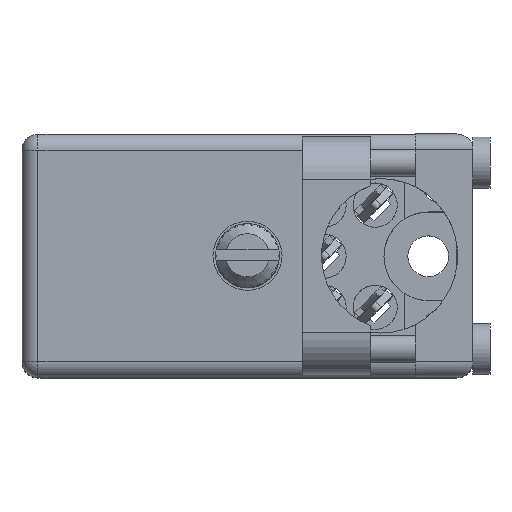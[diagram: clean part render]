
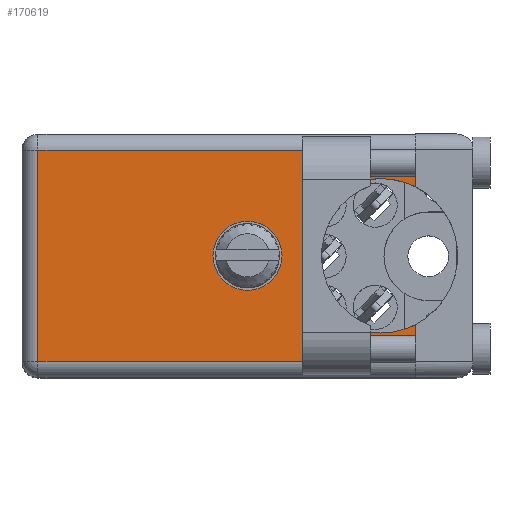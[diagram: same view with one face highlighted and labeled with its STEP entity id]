
A CAD part, top view. The second image highlights one B-rep face of the part: STEP entity #170619.
In plain terms, the highlighted face is planar.
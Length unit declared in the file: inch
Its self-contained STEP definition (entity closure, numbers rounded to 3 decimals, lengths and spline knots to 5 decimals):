
#3561 = AXIS2_PLACEMENT_3D ( 'NONE', #135737, #51711, #151351 ) ;
#6089 = ORIENTED_EDGE ( 'NONE', *, *, #53595, .F. ) ;
#8694 = LINE ( 'NONE', #50967, #156568 ) ;
#12902 = VECTOR ( 'NONE', #153332, 39.37008 ) ;
#13545 = ORIENTED_EDGE ( 'NONE', *, *, #129859, .F. ) ;
#19530 = CARTESIAN_POINT ( 'NONE',  ( 1.155, 0.906, -0.047 ) ) ;
#21340 = DIRECTION ( 'NONE',  ( 0., 1., 0. ) ) ;
#23151 = ORIENTED_EDGE ( 'NONE', *, *, #174199, .F. ) ;
#28073 = DIRECTION ( 'NONE',  ( 0., 0., 1. ) ) ;
#28147 = CARTESIAN_POINT ( 'NONE',  ( 1.155, 0.906, -0.047 ) ) ;
#28583 = AXIS2_PLACEMENT_3D ( 'NONE', #70898, #29603, #142340 ) ;
#29059 = DIRECTION ( 'NONE',  ( 0., 0., 1. ) ) ;
#29271 = CARTESIAN_POINT ( 'NONE',  ( 0.047, 0.906, -0.668 ) ) ;
#29603 = DIRECTION ( 'NONE',  ( 0., 1., 0. ) ) ;
#30458 = VERTEX_POINT ( 'NONE', #82985 ) ;
#31246 = AXIS2_PLACEMENT_3D ( 'NONE', #133064, #129263, #29059 ) ;
#33281 = DIRECTION ( 'NONE',  ( 0., 0., 1. ) ) ;
#36613 = DIRECTION ( 'NONE',  ( -1., 0., 0. ) ) ;
#39174 = EDGE_CURVE ( 'NONE', #137315, #173928, #170800, .T. ) ;
#39487 = LINE ( 'NONE', #28147, #147174 ) ;
#40610 = ORIENTED_EDGE ( 'NONE', *, *, #67839, .T. ) ;
#42143 = CIRCLE ( 'NONE', #3561, 0.1015 ) ;
#45993 = DIRECTION ( 'NONE',  ( 0., 0., 1. ) ) ;
#46814 = DIRECTION ( 'NONE',  ( 1., 0., 0. ) ) ;
#48871 = ORIENTED_EDGE ( 'NONE', *, *, #39174, .F. ) ;
#50967 = CARTESIAN_POINT ( 'NONE',  ( 0., 0.906, -0.668 ) ) ;
#51079 = AXIS2_PLACEMENT_3D ( 'NONE', #106501, #21340, #105235 ) ;
#51711 = DIRECTION ( 'NONE',  ( 0., 1., 0. ) ) ;
#53595 = EDGE_CURVE ( 'NONE', #85711, #162808, #42143, .T. ) ;
#54679 = EDGE_CURVE ( 'NONE', #141181, #30458, #125060, .T. ) ;
#54695 = CARTESIAN_POINT ( 'NONE',  ( 1.155, 0.906, 0. ) ) ;
#56258 = EDGE_CURVE ( 'NONE', #112871, #114663, #39487, .T. ) ;
#56536 = DIRECTION ( 'NONE',  ( 0., 0., 1. ) ) ;
#60198 = FACE_BOUND ( 'NONE', #161975, .T. ) ;
#62878 = ORIENTED_EDGE ( 'NONE', *, *, #135743, .F. ) ;
#63350 = VERTEX_POINT ( 'NONE', #29271 ) ;
#63875 = PLANE ( 'NONE',  #86470 ) ;
#64891 = CARTESIAN_POINT ( 'NONE',  ( 1.155, 0.906, -0.56029 ) ) ;
#67839 = EDGE_CURVE ( 'NONE', #112794, #63350, #8694, .T. ) ;
#69051 = ORIENTED_EDGE ( 'NONE', *, *, #54679, .F. ) ;
#70898 = CARTESIAN_POINT ( 'NONE',  ( 1.053, 0.906, -0.3575 ) ) ;
#80721 = ORIENTED_EDGE ( 'NONE', *, *, #147269, .T. ) ;
#82985 = CARTESIAN_POINT ( 'NONE',  ( 1.155, 0.906, -0.15471 ) ) ;
#85711 = VERTEX_POINT ( 'NONE', #140418 ) ;
#86129 = DIRECTION ( 'NONE',  ( 0., 1., 0. ) ) ;
#86470 = AXIS2_PLACEMENT_3D ( 'NONE', #105941, #162936, #33281 ) ;
#95079 = AXIS2_PLACEMENT_3D ( 'NONE', #171996, #86129, #45993 ) ;
#98975 = VECTOR ( 'NONE', #56536, 39.37008 ) ;
#105235 = DIRECTION ( 'NONE',  ( 0., 0., 1. ) ) ;
#105512 = CARTESIAN_POINT ( 'NONE',  ( 0.6625, 0.906, -0.256 ) ) ;
#105941 = CARTESIAN_POINT ( 'NONE',  ( 0., 0.906, -0.715 ) ) ;
#106501 = CARTESIAN_POINT ( 'NONE',  ( 0.6625, 0.906, -0.3575 ) ) ;
#109348 = CIRCLE ( 'NONE', #51079, 0.1015 ) ;
#112563 = EDGE_LOOP ( 'NONE', ( #160809, #40610, #80721, #170685, #62878, #69051, #13545, #48871 ) ) ;
#112794 = VERTEX_POINT ( 'NONE', #124601 ) ;
#112871 = VERTEX_POINT ( 'NONE', #147116 ) ;
#114663 = VERTEX_POINT ( 'NONE', #19530 ) ;
#122877 = CARTESIAN_POINT ( 'NONE',  ( 1.053, 0.906, -0.5845 ) ) ;
#124601 = CARTESIAN_POINT ( 'NONE',  ( 1.155, 0.906, -0.668 ) ) ;
#125060 = CIRCLE ( 'NONE', #31246, 0.227 ) ;
#127451 = EDGE_CURVE ( 'NONE', #112794, #137315, #167424, .T. ) ;
#129263 = DIRECTION ( 'NONE',  ( 0., 1., 0. ) ) ;
#129859 = EDGE_CURVE ( 'NONE', #173928, #141181, #169421, .T. ) ;
#133064 = CARTESIAN_POINT ( 'NONE',  ( 1.053, 0.906, -0.3575 ) ) ;
#135737 = CARTESIAN_POINT ( 'NONE',  ( 0.6625, 0.906, -0.3575 ) ) ;
#135743 = EDGE_CURVE ( 'NONE', #30458, #114663, #137105, .T. ) ;
#137105 = LINE ( 'NONE', #54695, #98975 ) ;
#137315 = VERTEX_POINT ( 'NONE', #64891 ) ;
#137987 = VECTOR ( 'NONE', #28073, 39.37008 ) ;
#140418 = CARTESIAN_POINT ( 'NONE',  ( 0.6625, 0.906, -0.459 ) ) ;
#141181 = VERTEX_POINT ( 'NONE', #148058 ) ;
#142340 = DIRECTION ( 'NONE',  ( 0., 0., 1. ) ) ;
#147116 = CARTESIAN_POINT ( 'NONE',  ( 0.047, 0.906, -0.047 ) ) ;
#147174 = VECTOR ( 'NONE', #46814, 39.37008 ) ;
#147269 = EDGE_CURVE ( 'NONE', #63350, #112871, #180654, .T. ) ;
#148058 = CARTESIAN_POINT ( 'NONE',  ( 1.053, 0.906, -0.1305 ) ) ;
#151351 = DIRECTION ( 'NONE',  ( 0., 0., 1. ) ) ;
#153332 = DIRECTION ( 'NONE',  ( 0., 0., 1. ) ) ;
#155188 = CARTESIAN_POINT ( 'NONE',  ( 0.047, 0.906, -0.715 ) ) ;
#156568 = VECTOR ( 'NONE', #36613, 39.37008 ) ;
#160809 = ORIENTED_EDGE ( 'NONE', *, *, #127451, .F. ) ;
#161975 = EDGE_LOOP ( 'NONE', ( #23151, #6089 ) ) ;
#162808 = VERTEX_POINT ( 'NONE', #105512 ) ;
#162936 = DIRECTION ( 'NONE',  ( 0., 1., 0. ) ) ;
#165556 = FACE_OUTER_BOUND ( 'NONE', #112563, .T. ) ;
#167424 = LINE ( 'NONE', #180385, #12902 ) ;
#169421 = CIRCLE ( 'NONE', #28583, 0.227 ) ;
#170619 = ADVANCED_FACE ( 'NONE', ( #165556, #60198 ), #63875, .T. ) ;
#170685 = ORIENTED_EDGE ( 'NONE', *, *, #56258, .T. ) ;
#170800 = CIRCLE ( 'NONE', #95079, 0.227 ) ;
#171996 = CARTESIAN_POINT ( 'NONE',  ( 1.053, 0.906, -0.3575 ) ) ;
#173928 = VERTEX_POINT ( 'NONE', #122877 ) ;
#174199 = EDGE_CURVE ( 'NONE', #162808, #85711, #109348, .T. ) ;
#180385 = CARTESIAN_POINT ( 'NONE',  ( 1.155, 0.906, 0. ) ) ;
#180654 = LINE ( 'NONE', #155188, #137987 ) ;
